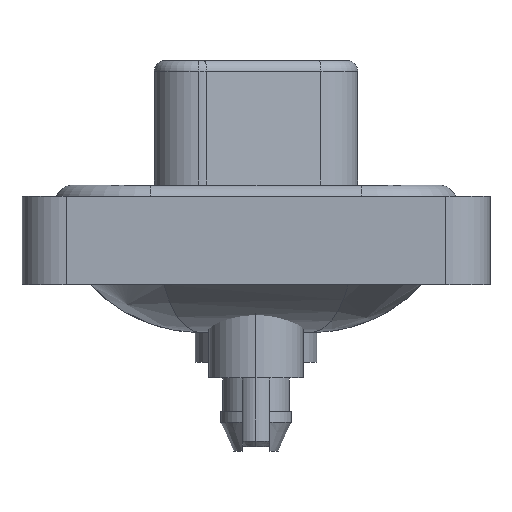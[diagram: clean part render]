
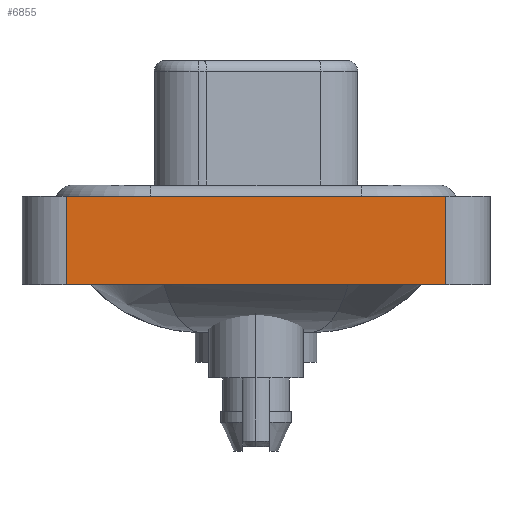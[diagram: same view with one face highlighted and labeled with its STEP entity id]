
A CAD part, left-side view. The second image highlights one B-rep face of the part: STEP entity #6855.
In plain terms, the highlighted planar face has unit normal (-1, 0, 0).
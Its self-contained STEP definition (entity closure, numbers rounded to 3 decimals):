
#1282 = VERTEX_POINT ( 'NONE', #7164 ) ;
#2944 = DIRECTION ( 'NONE',  ( 0., -1., 0. ) ) ;
#3221 = VECTOR ( 'NONE', #15062, 1000. ) ;
#3399 = ORIENTED_EDGE ( 'NONE', *, *, #4252, .F. ) ;
#4027 = VERTEX_POINT ( 'NONE', #8030 ) ;
#4215 = VERTEX_POINT ( 'NONE', #11555 ) ;
#4232 = CARTESIAN_POINT ( 'NONE',  ( -7.3, 8.55, -3.6 ) ) ;
#4252 = EDGE_CURVE ( 'NONE', #11079, #4027, #15402, .T. ) ;
#5835 = DIRECTION ( 'NONE',  ( 0., 0., 1. ) ) ;
#6855 = ADVANCED_FACE ( 'NONE', ( #9325 ), #11426, .T. ) ;
#7164 = CARTESIAN_POINT ( 'NONE',  ( -7.3, -8.55, -3.6 ) ) ;
#7249 = EDGE_LOOP ( 'NONE', ( #9162, #3399, #10440, #10353 ) ) ;
#8030 = CARTESIAN_POINT ( 'NONE',  ( -7.3, -8.55, 0.4 ) ) ;
#9162 = ORIENTED_EDGE ( 'NONE', *, *, #18996, .T. ) ;
#9325 = FACE_OUTER_BOUND ( 'NONE', #7249, .T. ) ;
#9732 = CARTESIAN_POINT ( 'NONE',  ( -7.3, 8.55, 0.4 ) ) ;
#9816 = DIRECTION ( 'NONE',  ( 0., 0., 1. ) ) ;
#10150 = AXIS2_PLACEMENT_3D ( 'NONE', #19148, #14290, #9816 ) ;
#10353 = ORIENTED_EDGE ( 'NONE', *, *, #12405, .T. ) ;
#10368 = VECTOR ( 'NONE', #2944, 1000. ) ;
#10440 = ORIENTED_EDGE ( 'NONE', *, *, #13159, .F. ) ;
#11079 = VERTEX_POINT ( 'NONE', #9732 ) ;
#11426 = PLANE ( 'NONE',  #10150 ) ;
#11555 = CARTESIAN_POINT ( 'NONE',  ( -7.3, 8.55, -3.6 ) ) ;
#11598 = VECTOR ( 'NONE', #5835, 1000. ) ;
#12151 = CARTESIAN_POINT ( 'NONE',  ( -7.3, -8.55, 0.4 ) ) ;
#12405 = EDGE_CURVE ( 'NONE', #4215, #1282, #15439, .T. ) ;
#13159 = EDGE_CURVE ( 'NONE', #4215, #11079, #18116, .T. ) ;
#14290 = DIRECTION ( 'NONE',  ( -1., 0., 0. ) ) ;
#15062 = DIRECTION ( 'NONE',  ( 0., 0., 1. ) ) ;
#15402 = LINE ( 'NONE', #12151, #10368 ) ;
#15439 = LINE ( 'NONE', #20002, #17779 ) ;
#15634 = DIRECTION ( 'NONE',  ( 0., -1., 0. ) ) ;
#16759 = CARTESIAN_POINT ( 'NONE',  ( -7.3, -8.55, -3.6 ) ) ;
#17779 = VECTOR ( 'NONE', #15634, 1000. ) ;
#18116 = LINE ( 'NONE', #4232, #3221 ) ;
#18384 = LINE ( 'NONE', #16759, #11598 ) ;
#18996 = EDGE_CURVE ( 'NONE', #1282, #4027, #18384, .T. ) ;
#19148 = CARTESIAN_POINT ( 'NONE',  ( -7.3, -8.55, -3.6 ) ) ;
#20002 = CARTESIAN_POINT ( 'NONE',  ( -7.3, -8.55, -3.6 ) ) ;
